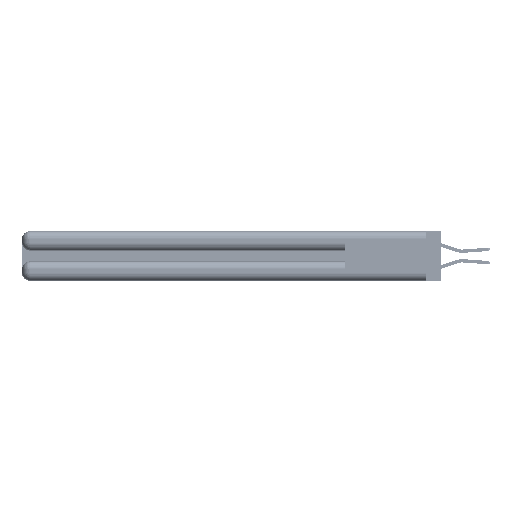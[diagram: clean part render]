
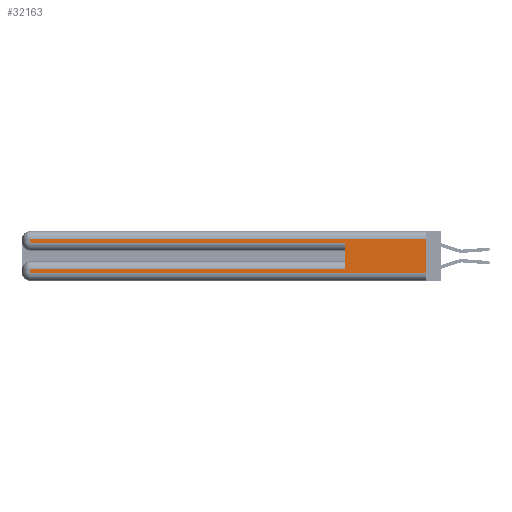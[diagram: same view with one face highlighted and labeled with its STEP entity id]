
A CAD part, left-side view. The second image highlights one B-rep face of the part: STEP entity #32163.
In plain terms, the highlighted planar face has unit normal (-1, 0, 0).
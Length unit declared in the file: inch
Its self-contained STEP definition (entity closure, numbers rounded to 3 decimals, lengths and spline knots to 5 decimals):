
#269 = VERTEX_POINT ( 'NONE', #39241 ) ;
#548 = DIRECTION ( 'NONE',  ( 0., 0., 1. ) ) ;
#1107 = VERTEX_POINT ( 'NONE', #35867 ) ;
#3681 = DIRECTION ( 'NONE',  ( 1., 0., 0. ) ) ;
#5112 = DIRECTION ( 'NONE',  ( 0., -1., 0. ) ) ;
#6203 = ORIENTED_EDGE ( 'NONE', *, *, #32706, .T. ) ;
#6464 = LINE ( 'NONE', #29934, #25096 ) ;
#6670 = CARTESIAN_POINT ( 'NONE',  ( 0., 2.94, 0.31 ) ) ;
#7557 = DIRECTION ( 'NONE',  ( 0., -1., 0. ) ) ;
#7793 = VECTOR ( 'NONE', #40625, 39.37008 ) ;
#9027 = LINE ( 'NONE', #28893, #7793 ) ;
#10682 = EDGE_CURVE ( 'NONE', #42673, #269, #9027, .T. ) ;
#10905 = VECTOR ( 'NONE', #5112, 39.37008 ) ;
#11142 = ORIENTED_EDGE ( 'NONE', *, *, #10682, .T. ) ;
#11146 = VECTOR ( 'NONE', #16394, 39.37008 ) ;
#11412 = CARTESIAN_POINT ( 'NONE',  ( 0., 0., 0.37 ) ) ;
#11653 = EDGE_CURVE ( 'NONE', #20716, #43515, #6464, .T. ) ;
#12140 = LINE ( 'NONE', #32880, #10905 ) ;
#12352 = CARTESIAN_POINT ( 'NONE',  ( 0., 0.6, 0.145 ) ) ;
#12820 = VECTOR ( 'NONE', #48027, 39.37008 ) ;
#15419 = DIRECTION ( 'NONE',  ( 0., 0., -1. ) ) ;
#16394 = DIRECTION ( 'NONE',  ( 0., 1., 0. ) ) ;
#18435 = EDGE_CURVE ( 'NONE', #19289, #1107, #20963, .T. ) ;
#19289 = VERTEX_POINT ( 'NONE', #32685 ) ;
#19857 = VERTEX_POINT ( 'NONE', #20286 ) ;
#20286 = CARTESIAN_POINT ( 'NONE',  ( 0., 0.6, 0.285 ) ) ;
#20465 = ORIENTED_EDGE ( 'NONE', *, *, #22248, .T. ) ;
#20535 = CARTESIAN_POINT ( 'NONE',  ( 0., 2.94, 0.285 ) ) ;
#20716 = VERTEX_POINT ( 'NONE', #6670 ) ;
#20963 = LINE ( 'NONE', #11412, #31535 ) ;
#21067 = EDGE_CURVE ( 'NONE', #269, #21270, #23397, .T. ) ;
#21270 = VERTEX_POINT ( 'NONE', #25716 ) ;
#22248 = EDGE_CURVE ( 'NONE', #21270, #1107, #29475, .T. ) ;
#22941 = LINE ( 'NONE', #44109, #11146 ) ;
#23397 = LINE ( 'NONE', #44042, #12820 ) ;
#25096 = VECTOR ( 'NONE', #33937, 39.37008 ) ;
#25716 = CARTESIAN_POINT ( 'NONE',  ( 0., 2.94, 0.06 ) ) ;
#26065 = VECTOR ( 'NONE', #548, 39.37008 ) ;
#27297 = LINE ( 'NONE', #12352, #26065 ) ;
#27508 = PLANE ( 'NONE',  #38673 ) ;
#28893 = CARTESIAN_POINT ( 'NONE',  ( 0., 0., 0.085 ) ) ;
#29475 = LINE ( 'NONE', #31321, #41199 ) ;
#29727 = ORIENTED_EDGE ( 'NONE', *, *, #21067, .T. ) ;
#29934 = CARTESIAN_POINT ( 'NONE',  ( 0., 2.94, 0.37 ) ) ;
#30527 = EDGE_CURVE ( 'NONE', #42673, #19857, #27297, .T. ) ;
#31300 = CARTESIAN_POINT ( 'NONE',  ( 0., 0., 0.37 ) ) ;
#31321 = CARTESIAN_POINT ( 'NONE',  ( 0., 0., 0.06 ) ) ;
#31474 = DIRECTION ( 'NONE',  ( 0., 0., -1. ) ) ;
#31535 = VECTOR ( 'NONE', #15419, 39.37008 ) ;
#32163 = ADVANCED_FACE ( 'NONE', ( #34567 ), #27508, .F. ) ;
#32685 = CARTESIAN_POINT ( 'NONE',  ( 0., 0., 0.31 ) ) ;
#32706 = EDGE_CURVE ( 'NONE', #43515, #19857, #12140, .T. ) ;
#32880 = CARTESIAN_POINT ( 'NONE',  ( 0., 0., 0.285 ) ) ;
#33937 = DIRECTION ( 'NONE',  ( 0., 0., -1. ) ) ;
#34567 = FACE_OUTER_BOUND ( 'NONE', #37248, .T. ) ;
#35867 = CARTESIAN_POINT ( 'NONE',  ( 0., 0., 0.06 ) ) ;
#36854 = ORIENTED_EDGE ( 'NONE', *, *, #30527, .F. ) ;
#37248 = EDGE_LOOP ( 'NONE', ( #47862, #47145, #43134, #6203, #36854, #11142, #29727, #20465 ) ) ;
#38673 = AXIS2_PLACEMENT_3D ( 'NONE', #31300, #3681, #31474 ) ;
#39241 = CARTESIAN_POINT ( 'NONE',  ( 0., 2.94, 0.085 ) ) ;
#39444 = EDGE_CURVE ( 'NONE', #19289, #20716, #22941, .T. ) ;
#40625 = DIRECTION ( 'NONE',  ( 0., 1., 0. ) ) ;
#41199 = VECTOR ( 'NONE', #7557, 39.37008 ) ;
#42673 = VERTEX_POINT ( 'NONE', #51287 ) ;
#43134 = ORIENTED_EDGE ( 'NONE', *, *, #11653, .T. ) ;
#43515 = VERTEX_POINT ( 'NONE', #20535 ) ;
#44042 = CARTESIAN_POINT ( 'NONE',  ( 0., 2.94, 0.37 ) ) ;
#44109 = CARTESIAN_POINT ( 'NONE',  ( 0., 0., 0.31 ) ) ;
#47145 = ORIENTED_EDGE ( 'NONE', *, *, #39444, .T. ) ;
#47862 = ORIENTED_EDGE ( 'NONE', *, *, #18435, .F. ) ;
#48027 = DIRECTION ( 'NONE',  ( 0., 0., -1. ) ) ;
#51287 = CARTESIAN_POINT ( 'NONE',  ( 0., 0.6, 0.085 ) ) ;
